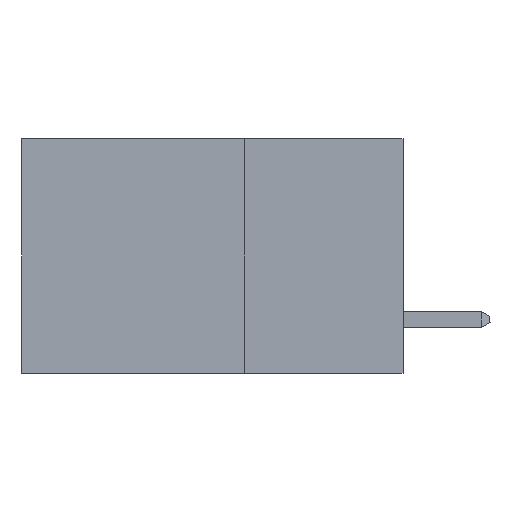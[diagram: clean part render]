
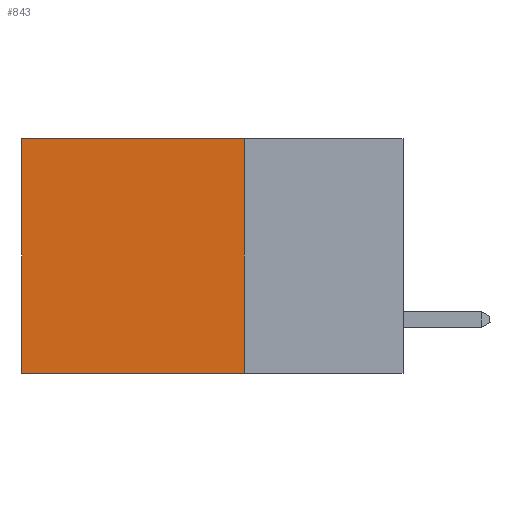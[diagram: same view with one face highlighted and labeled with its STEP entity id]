
A CAD part, left-side view. The second image highlights one B-rep face of the part: STEP entity #843.
In plain terms, the highlighted planar face has unit normal (-1, 0, 0).
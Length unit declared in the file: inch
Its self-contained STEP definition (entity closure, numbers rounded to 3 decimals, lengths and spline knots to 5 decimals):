
#178 = VERTEX_POINT ( 'NONE', #2879 ) ;
#301 = ORIENTED_EDGE ( 'NONE', *, *, #6330, .T. ) ;
#368 = FACE_OUTER_BOUND ( 'NONE', #6300, .T. ) ;
#843 = ADVANCED_FACE ( 'NONE', ( #368 ), #1663, .F. ) ;
#907 = LINE ( 'NONE', #8110, #6020 ) ;
#951 = LINE ( 'NONE', #3751, #4232 ) ;
#1282 = VERTEX_POINT ( 'NONE', #5982 ) ;
#1663 = PLANE ( 'NONE',  #4055 ) ;
#2643 = DIRECTION ( 'NONE',  ( 1., 0., 0. ) ) ;
#2876 = ORIENTED_EDGE ( 'NONE', *, *, #5263, .F. ) ;
#2879 = CARTESIAN_POINT ( 'NONE',  ( 0.2875, 0.6, -0.37 ) ) ;
#2905 = CARTESIAN_POINT ( 'NONE',  ( 0.2875, 0.25, -0.37 ) ) ;
#2973 = CARTESIAN_POINT ( 'NONE',  ( 0.2875, 0.25, -0.37 ) ) ;
#3751 = CARTESIAN_POINT ( 'NONE',  ( 0.2875, 0.6, 0. ) ) ;
#4055 = AXIS2_PLACEMENT_3D ( 'NONE', #9082, #2643, #13676 ) ;
#4232 = VECTOR ( 'NONE', #12216, 39.37008 ) ;
#4611 = DIRECTION ( 'NONE',  ( 0., 0., -1. ) ) ;
#5133 = VERTEX_POINT ( 'NONE', #7178 ) ;
#5263 = EDGE_CURVE ( 'NONE', #5133, #11827, #907, .T. ) ;
#5982 = CARTESIAN_POINT ( 'NONE',  ( 0.2875, 0.6, 0. ) ) ;
#6020 = VECTOR ( 'NONE', #4611, 39.37008 ) ;
#6300 = EDGE_LOOP ( 'NONE', ( #301, #12333, #2876, #9139 ) ) ;
#6330 = EDGE_CURVE ( 'NONE', #1282, #178, #951, .T. ) ;
#7069 = EDGE_CURVE ( 'NONE', #11827, #178, #8309, .T. ) ;
#7178 = CARTESIAN_POINT ( 'NONE',  ( 0.2875, 0.25, 0. ) ) ;
#7278 = LINE ( 'NONE', #11368, #12257 ) ;
#8110 = CARTESIAN_POINT ( 'NONE',  ( 0.2875, 0.25, 0. ) ) ;
#8309 = LINE ( 'NONE', #2905, #13678 ) ;
#9082 = CARTESIAN_POINT ( 'NONE',  ( 0.2875, 0.25, 0. ) ) ;
#9139 = ORIENTED_EDGE ( 'NONE', *, *, #10494, .T. ) ;
#10494 = EDGE_CURVE ( 'NONE', #5133, #1282, #7278, .T. ) ;
#11368 = CARTESIAN_POINT ( 'NONE',  ( 0.2875, 0.25, 0. ) ) ;
#11472 = DIRECTION ( 'NONE',  ( 0., 1., 0. ) ) ;
#11827 = VERTEX_POINT ( 'NONE', #2973 ) ;
#12216 = DIRECTION ( 'NONE',  ( 0., 0., -1. ) ) ;
#12257 = VECTOR ( 'NONE', #11472, 39.37008 ) ;
#12333 = ORIENTED_EDGE ( 'NONE', *, *, #7069, .F. ) ;
#13419 = DIRECTION ( 'NONE',  ( 0., 1., 0. ) ) ;
#13676 = DIRECTION ( 'NONE',  ( 0., 0., -1. ) ) ;
#13678 = VECTOR ( 'NONE', #13419, 39.37008 ) ;
